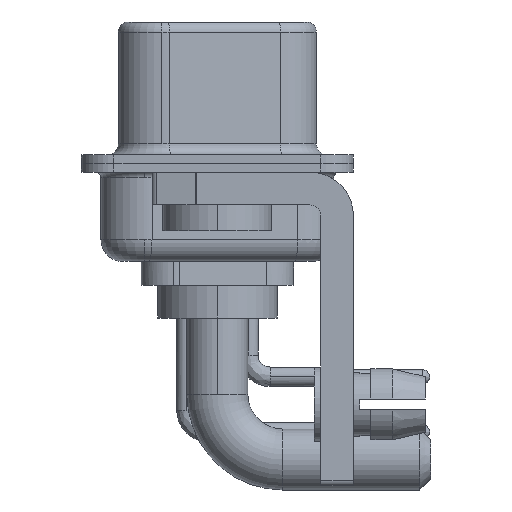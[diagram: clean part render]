
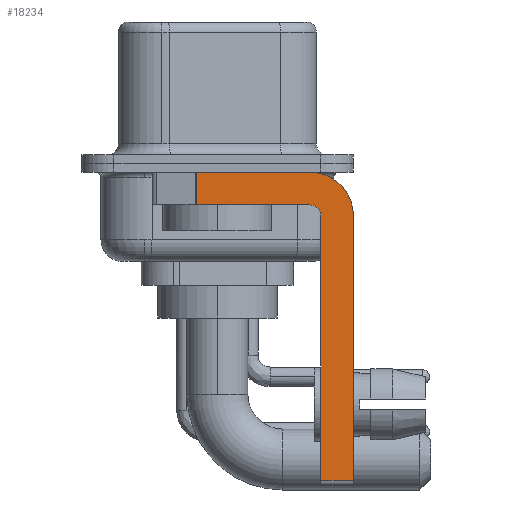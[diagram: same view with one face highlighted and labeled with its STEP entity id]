
A CAD part, left-side view. The second image highlights one B-rep face of the part: STEP entity #18234.
In plain terms, the highlighted planar face has unit normal (-1, 0, 0).
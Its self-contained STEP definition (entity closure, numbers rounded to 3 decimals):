
#304 = CARTESIAN_POINT ( 'NONE',  ( -2.9, 0.978, -0.4 ) ) ;
#403 = ORIENTED_EDGE ( 'NONE', *, *, #6919, .F. ) ;
#431 = ORIENTED_EDGE ( 'NONE', *, *, #22341, .F. ) ;
#563 = VECTOR ( 'NONE', #20369, 1000. ) ;
#587 = CARTESIAN_POINT ( 'NONE',  ( -2.9, -4.25, -14.55 ) ) ;
#721 = ORIENTED_EDGE ( 'NONE', *, *, #22339, .F. ) ;
#815 = DIRECTION ( 'NONE',  ( 0., -1., 0. ) ) ;
#888 = CARTESIAN_POINT ( 'NONE',  ( -2.9, -4.25, -1.9 ) ) ;
#962 = LINE ( 'NONE', #11687, #2776 ) ;
#1650 = VECTOR ( 'NONE', #20447, 1000. ) ;
#2198 = LINE ( 'NONE', #14691, #563 ) ;
#2497 = DIRECTION ( 'NONE',  ( 1., 0., 0. ) ) ;
#2547 = EDGE_LOOP ( 'NONE', ( #403, #19054, #17972, #15828, #431, #13536, #7042, #721 ) ) ;
#2776 = VECTOR ( 'NONE', #4432, 1000. ) ;
#3135 = VERTEX_POINT ( 'NONE', #304 ) ;
#3676 = DIRECTION ( 'NONE',  ( -1., 0., 0. ) ) ;
#4121 = LINE ( 'NONE', #888, #19339 ) ;
#4185 = AXIS2_PLACEMENT_3D ( 'NONE', #5958, #2497, #11780 ) ;
#4306 = AXIS2_PLACEMENT_3D ( 'NONE', #12955, #3676, #12474 ) ;
#4432 = DIRECTION ( 'NONE',  ( 0., 0., 1. ) ) ;
#4825 = CARTESIAN_POINT ( 'NONE',  ( -2.9, -4.75, -2.4 ) ) ;
#5395 = VERTEX_POINT ( 'NONE', #7043 ) ;
#5485 = EDGE_CURVE ( 'NONE', #5395, #21107, #18324, .T. ) ;
#5958 = CARTESIAN_POINT ( 'NONE',  ( -2.9, -4.25, -2.4 ) ) ;
#6186 = PLANE ( 'NONE',  #4185 ) ;
#6258 = DIRECTION ( 'NONE',  ( 0., 1., 0. ) ) ;
#6332 = DIRECTION ( 'NONE',  ( 1., 0., 0. ) ) ;
#6590 = CIRCLE ( 'NONE', #4306, 0.5 ) ;
#6910 = CARTESIAN_POINT ( 'NONE',  ( -2.9, 0.978, -1.9 ) ) ;
#6919 = EDGE_CURVE ( 'NONE', #3135, #23100, #2198, .T. ) ;
#7042 = ORIENTED_EDGE ( 'NONE', *, *, #5485, .F. ) ;
#7043 = CARTESIAN_POINT ( 'NONE',  ( -2.9, -6.25, -2.4 ) ) ;
#8335 = DIRECTION ( 'NONE',  ( 0., 0., -1. ) ) ;
#8845 = LINE ( 'NONE', #21785, #19577 ) ;
#9763 = FACE_OUTER_BOUND ( 'NONE', #2547, .T. ) ;
#9892 = EDGE_CURVE ( 'NONE', #3135, #10336, #8845, .T. ) ;
#10336 = VERTEX_POINT ( 'NONE', #6910 ) ;
#11406 = VECTOR ( 'NONE', #815, 1000. ) ;
#11491 = CARTESIAN_POINT ( 'NONE',  ( -2.9, -4.25, -0.4 ) ) ;
#11687 = CARTESIAN_POINT ( 'NONE',  ( -2.9, -4.75, -14.8 ) ) ;
#11780 = DIRECTION ( 'NONE',  ( 0., 0., -1. ) ) ;
#12474 = DIRECTION ( 'NONE',  ( 0., 0., 1. ) ) ;
#12955 = CARTESIAN_POINT ( 'NONE',  ( -2.9, -4.25, -2.4 ) ) ;
#13047 = AXIS2_PLACEMENT_3D ( 'NONE', #15694, #6332, #8335 ) ;
#13536 = ORIENTED_EDGE ( 'NONE', *, *, #18374, .T. ) ;
#14691 = CARTESIAN_POINT ( 'NONE',  ( -2.9, 3., -0.4 ) ) ;
#15694 = CARTESIAN_POINT ( 'NONE',  ( -2.9, -4.25, -2.4 ) ) ;
#15828 = ORIENTED_EDGE ( 'NONE', *, *, #21201, .F. ) ;
#16663 = CARTESIAN_POINT ( 'NONE',  ( -2.9, -6.25, -2.4 ) ) ;
#17633 = EDGE_CURVE ( 'NONE', #18449, #10336, #4121, .T. ) ;
#17721 = CARTESIAN_POINT ( 'NONE',  ( -2.9, -4.25, -1.9 ) ) ;
#17972 = ORIENTED_EDGE ( 'NONE', *, *, #17633, .F. ) ;
#18234 = ADVANCED_FACE ( 'NONE', ( #9763 ), #6186, .F. ) ;
#18324 = LINE ( 'NONE', #16663, #1650 ) ;
#18374 = EDGE_CURVE ( 'NONE', #19064, #21107, #18772, .T. ) ;
#18449 = VERTEX_POINT ( 'NONE', #17721 ) ;
#18752 = CARTESIAN_POINT ( 'NONE',  ( -2.9, -4.75, -14.55 ) ) ;
#18772 = LINE ( 'NONE', #587, #11406 ) ;
#19054 = ORIENTED_EDGE ( 'NONE', *, *, #9892, .T. ) ;
#19064 = VERTEX_POINT ( 'NONE', #18752 ) ;
#19339 = VECTOR ( 'NONE', #6258, 1000. ) ;
#19577 = VECTOR ( 'NONE', #20014, 1000. ) ;
#20014 = DIRECTION ( 'NONE',  ( 0., 0., -1. ) ) ;
#20369 = DIRECTION ( 'NONE',  ( 0., -1., 0. ) ) ;
#20447 = DIRECTION ( 'NONE',  ( 0., 0., -1. ) ) ;
#21088 = VERTEX_POINT ( 'NONE', #4825 ) ;
#21107 = VERTEX_POINT ( 'NONE', #21837 ) ;
#21201 = EDGE_CURVE ( 'NONE', #21088, #18449, #6590, .T. ) ;
#21785 = CARTESIAN_POINT ( 'NONE',  ( -2.9, 0.978, -1.9 ) ) ;
#21837 = CARTESIAN_POINT ( 'NONE',  ( -2.9, -6.25, -14.55 ) ) ;
#22339 = EDGE_CURVE ( 'NONE', #23100, #5395, #22853, .T. ) ;
#22341 = EDGE_CURVE ( 'NONE', #19064, #21088, #962, .T. ) ;
#22853 = CIRCLE ( 'NONE', #13047, 2. ) ;
#23100 = VERTEX_POINT ( 'NONE', #11491 ) ;
